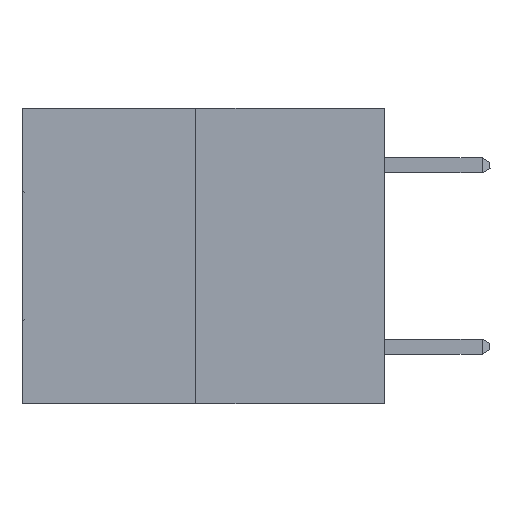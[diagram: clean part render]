
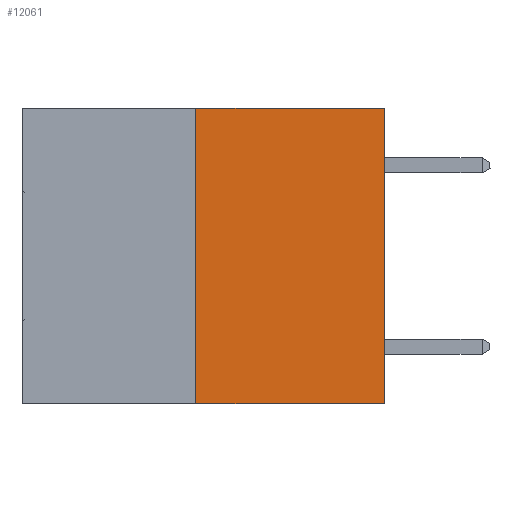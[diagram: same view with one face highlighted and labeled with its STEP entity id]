
A CAD part, left-side view. The second image highlights one B-rep face of the part: STEP entity #12061.
In plain terms, the highlighted planar face has unit normal (-1, 0, 0).
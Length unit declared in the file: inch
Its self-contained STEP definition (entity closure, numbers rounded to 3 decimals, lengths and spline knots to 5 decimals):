
#1434 = VECTOR ( 'NONE', #29291, 39.37008 ) ;
#1545 = LINE ( 'NONE', #28681, #23572 ) ;
#2578 = DIRECTION ( 'NONE',  ( 0., 0., 1. ) ) ;
#2952 = CARTESIAN_POINT ( 'NONE',  ( 0., 0.6, 0. ) ) ;
#3752 = VERTEX_POINT ( 'NONE', #18704 ) ;
#4241 = VECTOR ( 'NONE', #6506, 39.37008 ) ;
#5352 = ORIENTED_EDGE ( 'NONE', *, *, #11094, .T. ) ;
#5637 = DIRECTION ( 'NONE',  ( 1., 0., 0. ) ) ;
#6357 = VERTEX_POINT ( 'NONE', #23634 ) ;
#6506 = DIRECTION ( 'NONE',  ( 0., 0., 1. ) ) ;
#7948 = EDGE_CURVE ( 'NONE', #30922, #6357, #32507, .T. ) ;
#8636 = PLANE ( 'NONE',  #9223 ) ;
#9223 = AXIS2_PLACEMENT_3D ( 'NONE', #2952, #5637, #16503 ) ;
#11094 = EDGE_CURVE ( 'NONE', #30922, #3752, #1545, .T. ) ;
#11626 = EDGE_LOOP ( 'NONE', ( #33976, #5352, #25347, #20227 ) ) ;
#12061 = ADVANCED_FACE ( 'NONE', ( #15578 ), #8636, .F. ) ;
#12669 = VECTOR ( 'NONE', #2578, 39.37008 ) ;
#13048 = CARTESIAN_POINT ( 'NONE',  ( 0., 0., 0. ) ) ;
#13940 = LINE ( 'NONE', #15779, #12669 ) ;
#15578 = FACE_OUTER_BOUND ( 'NONE', #11626, .T. ) ;
#15779 = CARTESIAN_POINT ( 'NONE',  ( 0., 0., 0. ) ) ;
#15926 = LINE ( 'NONE', #26517, #1434 ) ;
#16087 = VERTEX_POINT ( 'NONE', #13048 ) ;
#16503 = DIRECTION ( 'NONE',  ( 0., 0., -1. ) ) ;
#18704 = CARTESIAN_POINT ( 'NONE',  ( 0., 0., -0.49 ) ) ;
#20227 = ORIENTED_EDGE ( 'NONE', *, *, #29919, .F. ) ;
#22451 = EDGE_CURVE ( 'NONE', #3752, #16087, #13940, .T. ) ;
#23572 = VECTOR ( 'NONE', #31260, 39.37008 ) ;
#23634 = CARTESIAN_POINT ( 'NONE',  ( 0., 0.312, 0. ) ) ;
#25347 = ORIENTED_EDGE ( 'NONE', *, *, #22451, .T. ) ;
#26517 = CARTESIAN_POINT ( 'NONE',  ( 0., 0.6, 0. ) ) ;
#28326 = CARTESIAN_POINT ( 'NONE',  ( 0., 0.312, -0.49 ) ) ;
#28681 = CARTESIAN_POINT ( 'NONE',  ( 0., 0.6, -0.49 ) ) ;
#29291 = DIRECTION ( 'NONE',  ( 0., -1., 0. ) ) ;
#29919 = EDGE_CURVE ( 'NONE', #6357, #16087, #15926, .T. ) ;
#30283 = CARTESIAN_POINT ( 'NONE',  ( 0., 0.312, -0.49 ) ) ;
#30922 = VERTEX_POINT ( 'NONE', #28326 ) ;
#31260 = DIRECTION ( 'NONE',  ( 0., -1., 0. ) ) ;
#32507 = LINE ( 'NONE', #30283, #4241 ) ;
#33976 = ORIENTED_EDGE ( 'NONE', *, *, #7948, .F. ) ;
